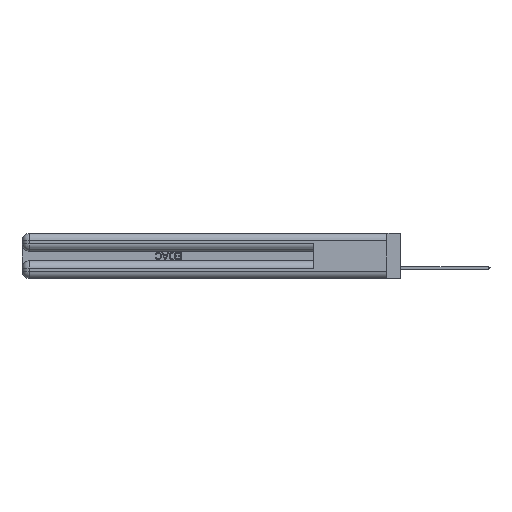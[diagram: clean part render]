
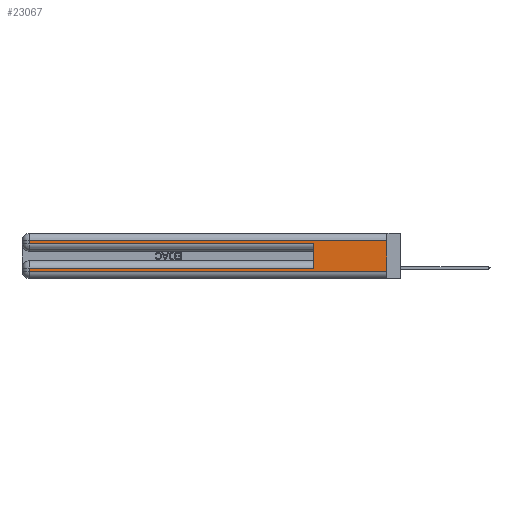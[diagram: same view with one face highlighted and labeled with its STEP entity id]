
A CAD part, left-side view. The second image highlights one B-rep face of the part: STEP entity #23067.
In plain terms, the highlighted planar face has unit normal (-1, 0, 0).
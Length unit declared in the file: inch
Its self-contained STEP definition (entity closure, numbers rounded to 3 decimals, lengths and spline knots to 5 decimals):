
#878 = CARTESIAN_POINT ( 'NONE',  ( 0., 0., 0.085 ) ) ;
#1777 = VECTOR ( 'NONE', #26842, 39.37008 ) ;
#1883 = VECTOR ( 'NONE', #11619, 39.37008 ) ;
#2196 = DIRECTION ( 'NONE',  ( 0., -1., 0. ) ) ;
#3822 = EDGE_CURVE ( 'NONE', #38502, #45843, #29195, .T. ) ;
#5862 = VECTOR ( 'NONE', #31849, 39.37008 ) ;
#7228 = DIRECTION ( 'NONE',  ( 1., 0., 0. ) ) ;
#7808 = VERTEX_POINT ( 'NONE', #15826 ) ;
#7890 = CARTESIAN_POINT ( 'NONE',  ( 0., 0.6, 0.085 ) ) ;
#9518 = CARTESIAN_POINT ( 'NONE',  ( 0., 0., 0.06 ) ) ;
#9820 = CARTESIAN_POINT ( 'NONE',  ( 0., 2.94, 0.31 ) ) ;
#9840 = ORIENTED_EDGE ( 'NONE', *, *, #31946, .T. ) ;
#9864 = CARTESIAN_POINT ( 'NONE',  ( 0., 0., 0.285 ) ) ;
#10197 = CARTESIAN_POINT ( 'NONE',  ( 0., 2.94, 0.37 ) ) ;
#10256 = FACE_OUTER_BOUND ( 'NONE', #11020, .T. ) ;
#10873 = CARTESIAN_POINT ( 'NONE',  ( 0., 2.94, 0.06 ) ) ;
#11020 = EDGE_LOOP ( 'NONE', ( #22473, #15836, #22538, #14350, #47836, #28703, #36091, #9840 ) ) ;
#11357 = VECTOR ( 'NONE', #46356, 39.37008 ) ;
#11619 = DIRECTION ( 'NONE',  ( 0., 0., -1. ) ) ;
#12174 = EDGE_CURVE ( 'NONE', #38410, #18335, #12479, .T. ) ;
#12479 = LINE ( 'NONE', #10197, #1883 ) ;
#12731 = EDGE_CURVE ( 'NONE', #24025, #45843, #47976, .T. ) ;
#13855 = DIRECTION ( 'NONE',  ( 0., -1., 0. ) ) ;
#14323 = VECTOR ( 'NONE', #2196, 39.37008 ) ;
#14350 = ORIENTED_EDGE ( 'NONE', *, *, #3822, .T. ) ;
#15826 = CARTESIAN_POINT ( 'NONE',  ( 0., 0., 0.06 ) ) ;
#15836 = ORIENTED_EDGE ( 'NONE', *, *, #37164, .T. ) ;
#15844 = CARTESIAN_POINT ( 'NONE',  ( 0., 0., 0.37 ) ) ;
#18335 = VERTEX_POINT ( 'NONE', #10873 ) ;
#18982 = DIRECTION ( 'NONE',  ( 0., 1., 0. ) ) ;
#21344 = VERTEX_POINT ( 'NONE', #38644 ) ;
#21500 = CARTESIAN_POINT ( 'NONE',  ( 0., 2.94, 0.285 ) ) ;
#21855 = CARTESIAN_POINT ( 'NONE',  ( 0., 2.94, 0.085 ) ) ;
#22473 = ORIENTED_EDGE ( 'NONE', *, *, #51598, .F. ) ;
#22538 = ORIENTED_EDGE ( 'NONE', *, *, #44484, .T. ) ;
#23067 = ADVANCED_FACE ( 'NONE', ( #10256 ), #38918, .F. ) ;
#23651 = VECTOR ( 'NONE', #13855, 39.37008 ) ;
#24025 = VERTEX_POINT ( 'NONE', #7890 ) ;
#26842 = DIRECTION ( 'NONE',  ( 0., 0., 1. ) ) ;
#27486 = EDGE_CURVE ( 'NONE', #24025, #38410, #39766, .T. ) ;
#28703 = ORIENTED_EDGE ( 'NONE', *, *, #27486, .T. ) ;
#28856 = LINE ( 'NONE', #15844, #5862 ) ;
#29195 = LINE ( 'NONE', #9864, #23651 ) ;
#30390 = VECTOR ( 'NONE', #48985, 39.37008 ) ;
#31849 = DIRECTION ( 'NONE',  ( 0., 0., -1. ) ) ;
#31946 = EDGE_CURVE ( 'NONE', #18335, #7808, #45571, .T. ) ;
#33366 = LINE ( 'NONE', #50707, #48405 ) ;
#34867 = CARTESIAN_POINT ( 'NONE',  ( 0., 0.6, 0.145 ) ) ;
#36091 = ORIENTED_EDGE ( 'NONE', *, *, #12174, .T. ) ;
#36849 = LINE ( 'NONE', #50129, #11357 ) ;
#37164 = EDGE_CURVE ( 'NONE', #21344, #39080, #33366, .T. ) ;
#38354 = CARTESIAN_POINT ( 'NONE',  ( 0., 0.6, 0.285 ) ) ;
#38410 = VERTEX_POINT ( 'NONE', #21855 ) ;
#38502 = VERTEX_POINT ( 'NONE', #21500 ) ;
#38644 = CARTESIAN_POINT ( 'NONE',  ( 0., 0., 0.31 ) ) ;
#38918 = PLANE ( 'NONE',  #43735 ) ;
#39080 = VERTEX_POINT ( 'NONE', #9820 ) ;
#39766 = LINE ( 'NONE', #878, #30390 ) ;
#43735 = AXIS2_PLACEMENT_3D ( 'NONE', #47652, #7228, #47156 ) ;
#44484 = EDGE_CURVE ( 'NONE', #39080, #38502, #36849, .T. ) ;
#45571 = LINE ( 'NONE', #9518, #14323 ) ;
#45843 = VERTEX_POINT ( 'NONE', #38354 ) ;
#46356 = DIRECTION ( 'NONE',  ( 0., 0., -1. ) ) ;
#47156 = DIRECTION ( 'NONE',  ( 0., 0., -1. ) ) ;
#47652 = CARTESIAN_POINT ( 'NONE',  ( 0., 0., 0.37 ) ) ;
#47836 = ORIENTED_EDGE ( 'NONE', *, *, #12731, .F. ) ;
#47976 = LINE ( 'NONE', #34867, #1777 ) ;
#48405 = VECTOR ( 'NONE', #18982, 39.37008 ) ;
#48985 = DIRECTION ( 'NONE',  ( 0., 1., 0. ) ) ;
#50129 = CARTESIAN_POINT ( 'NONE',  ( 0., 2.94, 0.37 ) ) ;
#50707 = CARTESIAN_POINT ( 'NONE',  ( 0., 0., 0.31 ) ) ;
#51598 = EDGE_CURVE ( 'NONE', #21344, #7808, #28856, .T. ) ;
